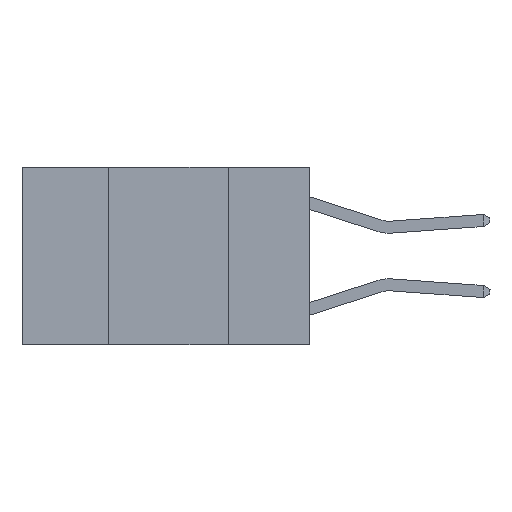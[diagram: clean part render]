
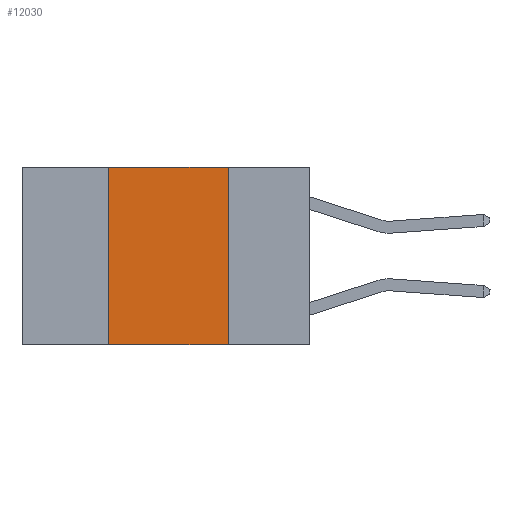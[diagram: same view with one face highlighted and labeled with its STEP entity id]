
A CAD part, left-side view. The second image highlights one B-rep face of the part: STEP entity #12030.
In plain terms, the highlighted planar face has unit normal (-1, 0, 0).
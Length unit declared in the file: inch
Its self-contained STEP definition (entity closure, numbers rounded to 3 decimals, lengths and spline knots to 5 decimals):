
#364 = PLANE ( 'NONE',  #870 ) ;
#754 = FACE_OUTER_BOUND ( 'NONE', #2787, .T. ) ;
#870 = AXIS2_PLACEMENT_3D ( 'NONE', #8734, #9924, #2773 ) ;
#1069 = VERTEX_POINT ( 'NONE', #4673 ) ;
#1185 = CARTESIAN_POINT ( 'NONE',  ( 0., 0.17, 0. ) ) ;
#2267 = LINE ( 'NONE', #5193, #5104 ) ;
#2297 = CARTESIAN_POINT ( 'NONE',  ( 0., 0.6, 0. ) ) ;
#2773 = DIRECTION ( 'NONE',  ( 0., 0., -1. ) ) ;
#2787 = EDGE_LOOP ( 'NONE', ( #8050, #14282, #14651, #15028 ) ) ;
#3076 = DIRECTION ( 'NONE',  ( 0., 0., -1. ) ) ;
#3507 = DIRECTION ( 'NONE',  ( 0., -1., 0. ) ) ;
#3603 = VECTOR ( 'NONE', #13767, 39.37008 ) ;
#3983 = LINE ( 'NONE', #11419, #9960 ) ;
#4673 = CARTESIAN_POINT ( 'NONE',  ( 0., 0.17, -0.37 ) ) ;
#5104 = VECTOR ( 'NONE', #6390, 39.37008 ) ;
#5113 = VERTEX_POINT ( 'NONE', #12239 ) ;
#5148 = EDGE_CURVE ( 'NONE', #7443, #5113, #2267, .T. ) ;
#5193 = CARTESIAN_POINT ( 'NONE',  ( 0., 0.42, 0. ) ) ;
#5693 = CARTESIAN_POINT ( 'NONE',  ( 0., 0.42, -0.37 ) ) ;
#6390 = DIRECTION ( 'NONE',  ( 0., 0., 1. ) ) ;
#7443 = VERTEX_POINT ( 'NONE', #5693 ) ;
#7549 = LINE ( 'NONE', #12579, #3603 ) ;
#7570 = LINE ( 'NONE', #2297, #12003 ) ;
#8050 = ORIENTED_EDGE ( 'NONE', *, *, #14615, .F. ) ;
#8734 = CARTESIAN_POINT ( 'NONE',  ( 0., 0.6, 0. ) ) ;
#9857 = EDGE_CURVE ( 'NONE', #5113, #11870, #7570, .T. ) ;
#9924 = DIRECTION ( 'NONE',  ( 1., 0., 0. ) ) ;
#9960 = VECTOR ( 'NONE', #3076, 39.37008 ) ;
#11419 = CARTESIAN_POINT ( 'NONE',  ( 0., 0.17, 0. ) ) ;
#11870 = VERTEX_POINT ( 'NONE', #1185 ) ;
#12003 = VECTOR ( 'NONE', #3507, 39.37008 ) ;
#12030 = ADVANCED_FACE ( 'NONE', ( #754 ), #364, .F. ) ;
#12239 = CARTESIAN_POINT ( 'NONE',  ( 0., 0.42, 0. ) ) ;
#12579 = CARTESIAN_POINT ( 'NONE',  ( 0., 0.6, -0.37 ) ) ;
#13767 = DIRECTION ( 'NONE',  ( 0., -1., 0. ) ) ;
#14282 = ORIENTED_EDGE ( 'NONE', *, *, #9857, .F. ) ;
#14615 = EDGE_CURVE ( 'NONE', #11870, #1069, #3983, .T. ) ;
#14617 = EDGE_CURVE ( 'NONE', #7443, #1069, #7549, .T. ) ;
#14651 = ORIENTED_EDGE ( 'NONE', *, *, #5148, .F. ) ;
#15028 = ORIENTED_EDGE ( 'NONE', *, *, #14617, .T. ) ;
